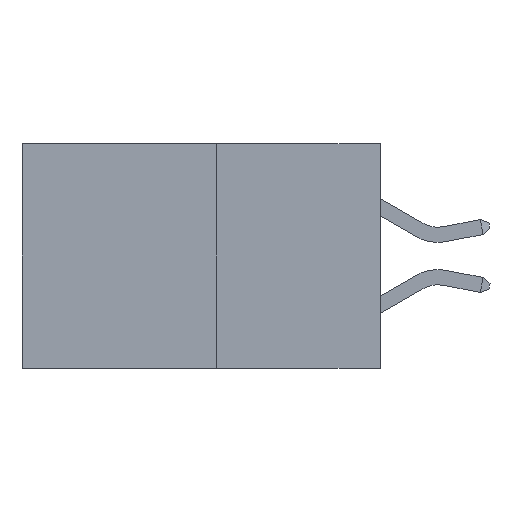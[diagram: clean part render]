
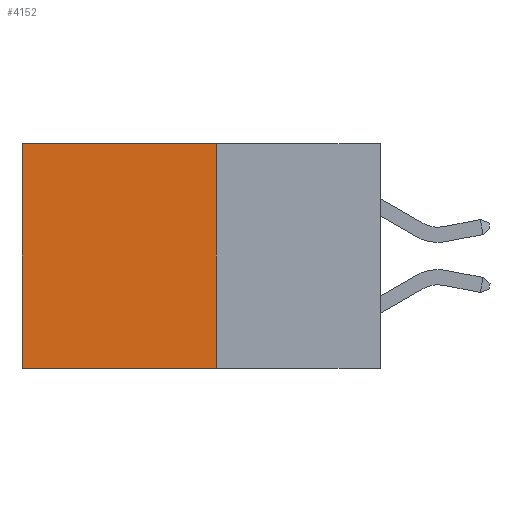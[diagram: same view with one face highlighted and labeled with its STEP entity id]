
A CAD part, left-side view. The second image highlights one B-rep face of the part: STEP entity #4152.
In plain terms, the highlighted planar face has unit normal (-1, 0, 0).
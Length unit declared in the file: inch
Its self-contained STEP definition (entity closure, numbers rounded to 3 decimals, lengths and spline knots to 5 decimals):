
#138 = VERTEX_POINT ( 'NONE', #7452 ) ;
#302 = VECTOR ( 'NONE', #1950, 39.37008 ) ;
#468 = CARTESIAN_POINT ( 'NONE',  ( 0.277, 0.59, 0. ) ) ;
#1282 = ORIENTED_EDGE ( 'NONE', *, *, #2939, .F. ) ;
#1307 = CARTESIAN_POINT ( 'NONE',  ( 0.277, 0.59, -0.37 ) ) ;
#1348 = VERTEX_POINT ( 'NONE', #468 ) ;
#1397 = LINE ( 'NONE', #7122, #4438 ) ;
#1662 = VERTEX_POINT ( 'NONE', #1307 ) ;
#1678 = CARTESIAN_POINT ( 'NONE',  ( 0.277, 0.59, -0.37 ) ) ;
#1950 = DIRECTION ( 'NONE',  ( 0., 1., 0. ) ) ;
#2308 = DIRECTION ( 'NONE',  ( 0., 0., -1. ) ) ;
#2536 = CARTESIAN_POINT ( 'NONE',  ( 0.277, 0.27, 0. ) ) ;
#2673 = DIRECTION ( 'NONE',  ( 0., 1., 0. ) ) ;
#2939 = EDGE_CURVE ( 'NONE', #4860, #138, #1397, .T. ) ;
#3077 = LINE ( 'NONE', #6526, #6093 ) ;
#3081 = AXIS2_PLACEMENT_3D ( 'NONE', #5084, #5188, #5156 ) ;
#3209 = EDGE_LOOP ( 'NONE', ( #3906, #7172, #1282, #5206 ) ) ;
#3601 = LINE ( 'NONE', #1678, #6820 ) ;
#3769 = EDGE_CURVE ( 'NONE', #138, #1662, #5575, .T. ) ;
#3906 = ORIENTED_EDGE ( 'NONE', *, *, #6057, .T. ) ;
#4152 = ADVANCED_FACE ( 'NONE', ( #5947 ), #4492, .F. ) ;
#4438 = VECTOR ( 'NONE', #6661, 39.37008 ) ;
#4492 = PLANE ( 'NONE',  #3081 ) ;
#4860 = VERTEX_POINT ( 'NONE', #2536 ) ;
#5084 = CARTESIAN_POINT ( 'NONE',  ( 0.277, 0.27, -0.37 ) ) ;
#5156 = DIRECTION ( 'NONE',  ( 0., 0., -1. ) ) ;
#5188 = DIRECTION ( 'NONE',  ( 1., 0., 0. ) ) ;
#5206 = ORIENTED_EDGE ( 'NONE', *, *, #7522, .T. ) ;
#5575 = LINE ( 'NONE', #5811, #302 ) ;
#5811 = CARTESIAN_POINT ( 'NONE',  ( 0.277, 0.27, -0.37 ) ) ;
#5947 = FACE_OUTER_BOUND ( 'NONE', #3209, .T. ) ;
#6057 = EDGE_CURVE ( 'NONE', #1348, #1662, #3601, .T. ) ;
#6093 = VECTOR ( 'NONE', #2673, 39.37008 ) ;
#6526 = CARTESIAN_POINT ( 'NONE',  ( 0.277, 0.27, 0. ) ) ;
#6661 = DIRECTION ( 'NONE',  ( 0., 0., -1. ) ) ;
#6820 = VECTOR ( 'NONE', #2308, 39.37008 ) ;
#7122 = CARTESIAN_POINT ( 'NONE',  ( 0.277, 0.27, -0.37 ) ) ;
#7172 = ORIENTED_EDGE ( 'NONE', *, *, #3769, .F. ) ;
#7452 = CARTESIAN_POINT ( 'NONE',  ( 0.277, 0.27, -0.37 ) ) ;
#7522 = EDGE_CURVE ( 'NONE', #4860, #1348, #3077, .T. ) ;
